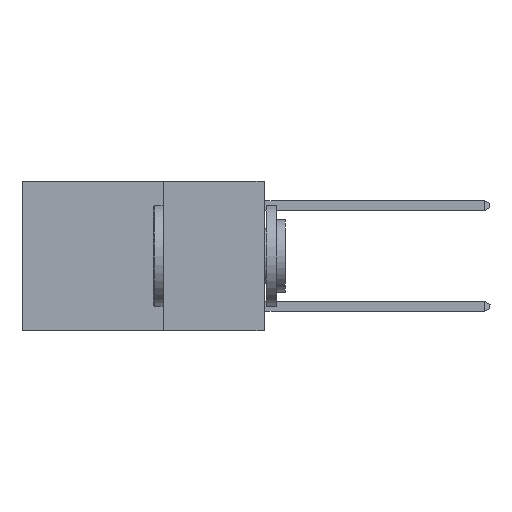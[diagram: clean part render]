
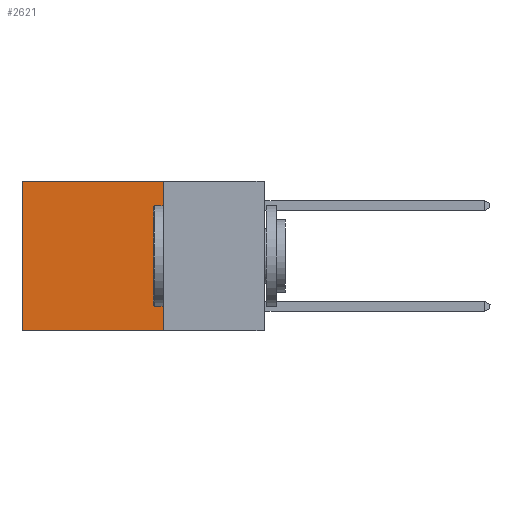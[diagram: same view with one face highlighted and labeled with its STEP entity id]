
A CAD part, left-side view. The second image highlights one B-rep face of the part: STEP entity #2621.
In plain terms, the highlighted planar face has unit normal (-1, 0, 0).
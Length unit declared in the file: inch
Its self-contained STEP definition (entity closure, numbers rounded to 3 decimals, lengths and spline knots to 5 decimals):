
#67 = CARTESIAN_POINT ( 'NONE',  ( 0.2625, 0.6, 0. ) ) ;
#1165 = CARTESIAN_POINT ( 'NONE',  ( 0.2625, 0.25, 0. ) ) ;
#1484 = CARTESIAN_POINT ( 'NONE',  ( 0.2625, 0.6, 0. ) ) ;
#1576 = DIRECTION ( 'NONE',  ( 0., 0., -1. ) ) ;
#1603 = VECTOR ( 'NONE', #6233, 39.37008 ) ;
#1754 = CARTESIAN_POINT ( 'NONE',  ( 0.2625, 0.25, 0. ) ) ;
#1815 = DIRECTION ( 'NONE',  ( 1., 0., 0. ) ) ;
#2057 = VECTOR ( 'NONE', #4835, 39.37008 ) ;
#2302 = VECTOR ( 'NONE', #9845, 39.37008 ) ;
#2384 = VECTOR ( 'NONE', #1576, 39.37008 ) ;
#2431 = AXIS2_PLACEMENT_3D ( 'NONE', #1754, #1815, #4154 ) ;
#2621 = ADVANCED_FACE ( 'NONE', ( #7603 ), #3329, .F. ) ;
#2807 = ORIENTED_EDGE ( 'NONE', *, *, #8751, .T. ) ;
#2822 = VERTEX_POINT ( 'NONE', #4535 ) ;
#3073 = EDGE_CURVE ( 'NONE', #9766, #2822, #7842, .T. ) ;
#3329 = PLANE ( 'NONE',  #2431 ) ;
#3532 = VERTEX_POINT ( 'NONE', #9642 ) ;
#3971 = EDGE_CURVE ( 'NONE', #8748, #2822, #6901, .T. ) ;
#4120 = EDGE_CURVE ( 'NONE', #3532, #8748, #8438, .T. ) ;
#4154 = DIRECTION ( 'NONE',  ( 0., 0., -1. ) ) ;
#4460 = ORIENTED_EDGE ( 'NONE', *, *, #3971, .F. ) ;
#4535 = CARTESIAN_POINT ( 'NONE',  ( 0.2625, 0.6, -0.37 ) ) ;
#4769 = EDGE_LOOP ( 'NONE', ( #5706, #4460, #4966, #2807 ) ) ;
#4835 = DIRECTION ( 'NONE',  ( 0., 1., 0. ) ) ;
#4966 = ORIENTED_EDGE ( 'NONE', *, *, #4120, .F. ) ;
#5706 = ORIENTED_EDGE ( 'NONE', *, *, #3073, .T. ) ;
#6233 = DIRECTION ( 'NONE',  ( 0., 0., -1. ) ) ;
#6901 = LINE ( 'NONE', #8108, #2302 ) ;
#7266 = CARTESIAN_POINT ( 'NONE',  ( 0.2625, 0.25, 0. ) ) ;
#7603 = FACE_OUTER_BOUND ( 'NONE', #4769, .T. ) ;
#7842 = LINE ( 'NONE', #1484, #2384 ) ;
#8053 = CARTESIAN_POINT ( 'NONE',  ( 0.2625, 0.25, -0.37 ) ) ;
#8108 = CARTESIAN_POINT ( 'NONE',  ( 0.2625, 0.25, -0.37 ) ) ;
#8438 = LINE ( 'NONE', #1165, #1603 ) ;
#8748 = VERTEX_POINT ( 'NONE', #8053 ) ;
#8751 = EDGE_CURVE ( 'NONE', #3532, #9766, #10441, .T. ) ;
#9642 = CARTESIAN_POINT ( 'NONE',  ( 0.2625, 0.25, 0. ) ) ;
#9766 = VERTEX_POINT ( 'NONE', #67 ) ;
#9845 = DIRECTION ( 'NONE',  ( 0., 1., 0. ) ) ;
#10441 = LINE ( 'NONE', #7266, #2057 ) ;
